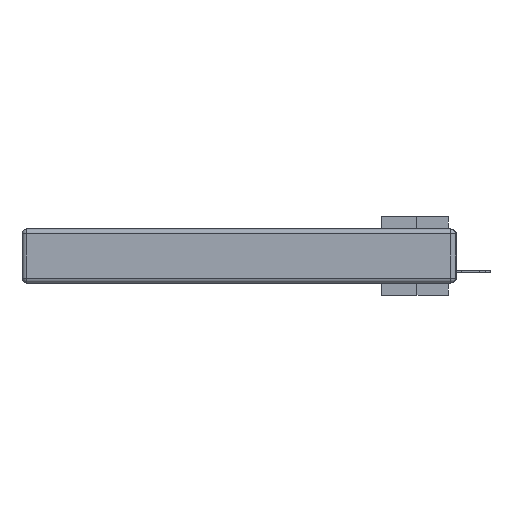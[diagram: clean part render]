
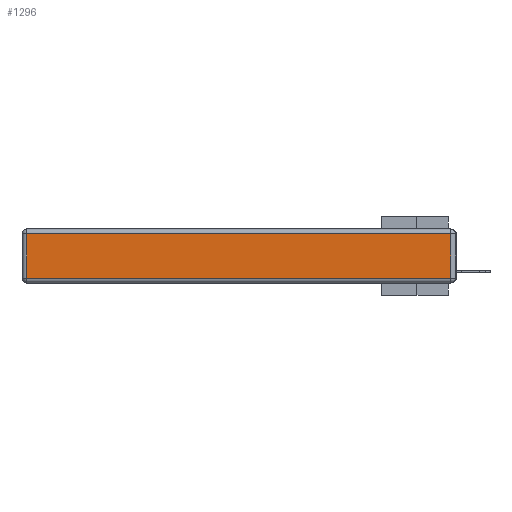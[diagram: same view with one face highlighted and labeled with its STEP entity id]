
A CAD part, left-side view. The second image highlights one B-rep face of the part: STEP entity #1296.
In plain terms, the highlighted planar face has unit normal (-1, 0, 0).
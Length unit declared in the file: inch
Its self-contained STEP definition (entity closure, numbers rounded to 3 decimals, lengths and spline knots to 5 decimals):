
#279 = CARTESIAN_POINT ( 'NONE',  ( 0., 0.03, -0.313 ) ) ;
#953 = EDGE_CURVE ( 'NONE', #20633, #2578, #27196, .T. ) ;
#1296 = ADVANCED_FACE ( 'NONE', ( #7742 ), #23883, .T. ) ;
#1513 = CARTESIAN_POINT ( 'NONE',  ( 0., 0., -0.343 ) ) ;
#1617 = LINE ( 'NONE', #12090, #23722 ) ;
#2578 = VERTEX_POINT ( 'NONE', #4939 ) ;
#2590 = ORIENTED_EDGE ( 'NONE', *, *, #28955, .T. ) ;
#3700 = VERTEX_POINT ( 'NONE', #29712 ) ;
#4939 = CARTESIAN_POINT ( 'NONE',  ( 0., 2.72, -0.313 ) ) ;
#7659 = ORIENTED_EDGE ( 'NONE', *, *, #953, .T. ) ;
#7742 = FACE_OUTER_BOUND ( 'NONE', #25881, .T. ) ;
#7795 = VECTOR ( 'NONE', #13545, 39.37008 ) ;
#8902 = DIRECTION ( 'NONE',  ( -1., 0., 0. ) ) ;
#11691 = DIRECTION ( 'NONE',  ( 0., 0., 1. ) ) ;
#12090 = CARTESIAN_POINT ( 'NONE',  ( 0., 0.03, -0.343 ) ) ;
#13545 = DIRECTION ( 'NONE',  ( 0., 1., 0. ) ) ;
#14128 = EDGE_CURVE ( 'NONE', #3700, #20633, #19546, .T. ) ;
#15142 = VECTOR ( 'NONE', #31135, 39.37008 ) ;
#15260 = ORIENTED_EDGE ( 'NONE', *, *, #24852, .T. ) ;
#16964 = VECTOR ( 'NONE', #17903, 39.37008 ) ;
#17903 = DIRECTION ( 'NONE',  ( 0., 0., -1. ) ) ;
#18556 = DIRECTION ( 'NONE',  ( 0., 0., 1. ) ) ;
#18948 = LINE ( 'NONE', #29108, #15142 ) ;
#18995 = VERTEX_POINT ( 'NONE', #279 ) ;
#19546 = LINE ( 'NONE', #28096, #7795 ) ;
#20633 = VERTEX_POINT ( 'NONE', #23284 ) ;
#22707 = AXIS2_PLACEMENT_3D ( 'NONE', #1513, #8902, #18556 ) ;
#23284 = CARTESIAN_POINT ( 'NONE',  ( 0., 2.72, -0.03 ) ) ;
#23683 = ORIENTED_EDGE ( 'NONE', *, *, #14128, .T. ) ;
#23722 = VECTOR ( 'NONE', #11691, 39.37008 ) ;
#23883 = PLANE ( 'NONE',  #22707 ) ;
#24852 = EDGE_CURVE ( 'NONE', #2578, #18995, #18948, .T. ) ;
#25881 = EDGE_LOOP ( 'NONE', ( #15260, #2590, #23683, #7659 ) ) ;
#26830 = CARTESIAN_POINT ( 'NONE',  ( 0., 2.72, -0.343 ) ) ;
#27196 = LINE ( 'NONE', #26830, #16964 ) ;
#28096 = CARTESIAN_POINT ( 'NONE',  ( 0., 2.75, -0.03 ) ) ;
#28955 = EDGE_CURVE ( 'NONE', #18995, #3700, #1617, .T. ) ;
#29108 = CARTESIAN_POINT ( 'NONE',  ( 0., 0., -0.313 ) ) ;
#29712 = CARTESIAN_POINT ( 'NONE',  ( 0., 0.03, -0.03 ) ) ;
#31135 = DIRECTION ( 'NONE',  ( 0., -1., 0. ) ) ;
